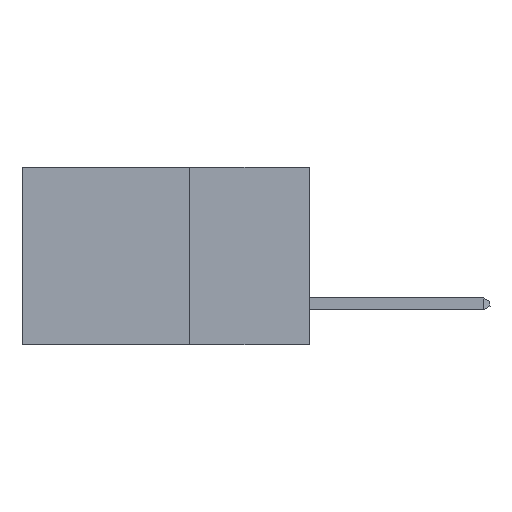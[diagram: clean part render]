
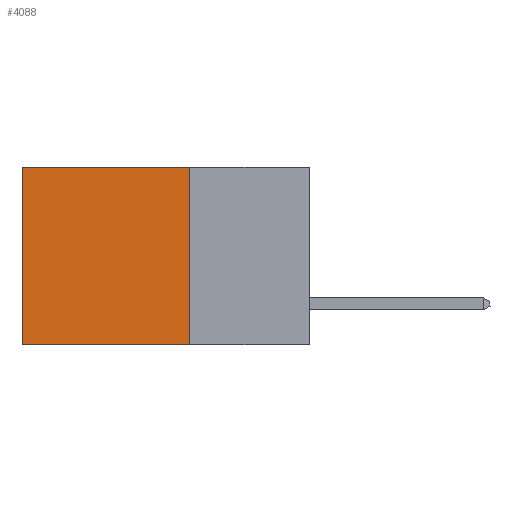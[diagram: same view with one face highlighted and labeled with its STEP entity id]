
A CAD part, left-side view. The second image highlights one B-rep face of the part: STEP entity #4088.
In plain terms, the highlighted planar face has unit normal (-1, 0, 0).
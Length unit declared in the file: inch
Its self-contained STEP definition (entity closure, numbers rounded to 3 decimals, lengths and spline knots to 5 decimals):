
#75 = EDGE_CURVE ( 'NONE', #1724, #1114, #2209, .T. ) ;
#311 = FACE_OUTER_BOUND ( 'NONE', #1094, .T. ) ;
#573 = AXIS2_PLACEMENT_3D ( 'NONE', #3749, #5138, #17236 ) ;
#598 = DIRECTION ( 'NONE',  ( 0., 0., -1. ) ) ;
#600 = VECTOR ( 'NONE', #2190, 39.37008 ) ;
#1094 = EDGE_LOOP ( 'NONE', ( #6287, #9846, #6142, #16725 ) ) ;
#1114 = VERTEX_POINT ( 'NONE', #8277 ) ;
#1482 = CARTESIAN_POINT ( 'NONE',  ( 0.2875, 0.6, 0. ) ) ;
#1724 = VERTEX_POINT ( 'NONE', #5010 ) ;
#1898 = EDGE_CURVE ( 'NONE', #1114, #16444, #4166, .T. ) ;
#2190 = DIRECTION ( 'NONE',  ( 0., 1., 0. ) ) ;
#2209 = LINE ( 'NONE', #7083, #15884 ) ;
#3212 = LINE ( 'NONE', #4046, #16456 ) ;
#3749 = CARTESIAN_POINT ( 'NONE',  ( 0.2875, 0.25, 0. ) ) ;
#3802 = PLANE ( 'NONE',  #573 ) ;
#4046 = CARTESIAN_POINT ( 'NONE',  ( 0.2875, 0.25, 0. ) ) ;
#4088 = ADVANCED_FACE ( 'NONE', ( #311 ), #3802, .F. ) ;
#4094 = DIRECTION ( 'NONE',  ( 0., 1., 0. ) ) ;
#4166 = LINE ( 'NONE', #12939, #600 ) ;
#4665 = VERTEX_POINT ( 'NONE', #1482 ) ;
#5010 = CARTESIAN_POINT ( 'NONE',  ( 0.2875, 0.25, 0. ) ) ;
#5138 = DIRECTION ( 'NONE',  ( 1., 0., 0. ) ) ;
#6047 = DIRECTION ( 'NONE',  ( 0., 0., -1. ) ) ;
#6142 = ORIENTED_EDGE ( 'NONE', *, *, #75, .F. ) ;
#6287 = ORIENTED_EDGE ( 'NONE', *, *, #9214, .T. ) ;
#7083 = CARTESIAN_POINT ( 'NONE',  ( 0.2875, 0.25, 0. ) ) ;
#8277 = CARTESIAN_POINT ( 'NONE',  ( 0.2875, 0.25, -0.37 ) ) ;
#9214 = EDGE_CURVE ( 'NONE', #4665, #16444, #12907, .T. ) ;
#9846 = ORIENTED_EDGE ( 'NONE', *, *, #1898, .F. ) ;
#12483 = VECTOR ( 'NONE', #598, 39.37008 ) ;
#12907 = LINE ( 'NONE', #13906, #12483 ) ;
#12939 = CARTESIAN_POINT ( 'NONE',  ( 0.2875, 0.25, -0.37 ) ) ;
#13906 = CARTESIAN_POINT ( 'NONE',  ( 0.2875, 0.6, 0. ) ) ;
#14406 = CARTESIAN_POINT ( 'NONE',  ( 0.2875, 0.6, -0.37 ) ) ;
#15848 = EDGE_CURVE ( 'NONE', #1724, #4665, #3212, .T. ) ;
#15884 = VECTOR ( 'NONE', #6047, 39.37008 ) ;
#16444 = VERTEX_POINT ( 'NONE', #14406 ) ;
#16456 = VECTOR ( 'NONE', #4094, 39.37008 ) ;
#16725 = ORIENTED_EDGE ( 'NONE', *, *, #15848, .T. ) ;
#17236 = DIRECTION ( 'NONE',  ( 0., 0., -1. ) ) ;
